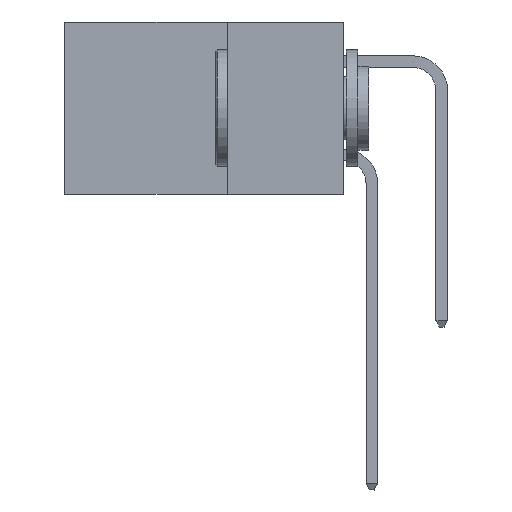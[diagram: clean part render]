
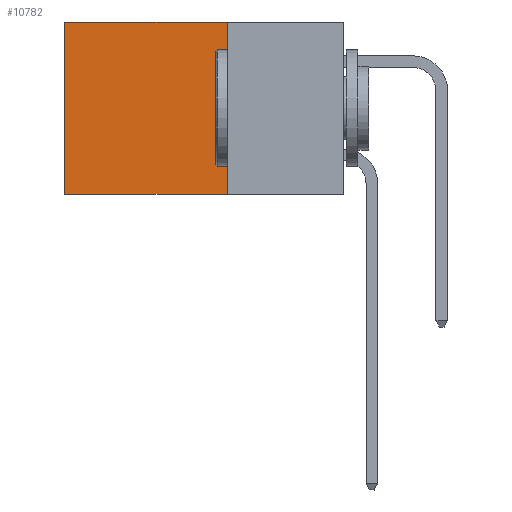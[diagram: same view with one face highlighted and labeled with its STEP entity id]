
A CAD part, left-side view. The second image highlights one B-rep face of the part: STEP entity #10782.
In plain terms, the highlighted planar face has unit normal (-1, 0, 0).
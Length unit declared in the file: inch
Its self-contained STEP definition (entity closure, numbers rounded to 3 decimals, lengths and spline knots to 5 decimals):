
#31 = ORIENTED_EDGE ( 'NONE', *, *, #5547, .F. ) ;
#980 = VERTEX_POINT ( 'NONE', #5932 ) ;
#2408 = LINE ( 'NONE', #18293, #6384 ) ;
#2844 = ORIENTED_EDGE ( 'NONE', *, *, #20150, .T. ) ;
#3345 = LINE ( 'NONE', #13109, #7808 ) ;
#3362 = DIRECTION ( 'NONE',  ( 0., 1., 0. ) ) ;
#3739 = VERTEX_POINT ( 'NONE', #16161 ) ;
#3865 = CARTESIAN_POINT ( 'NONE',  ( 0.298, 0.25, -0.37 ) ) ;
#3930 = LINE ( 'NONE', #16049, #13064 ) ;
#4838 = DIRECTION ( 'NONE',  ( 1., 0., 0. ) ) ;
#5547 = EDGE_CURVE ( 'NONE', #10440, #3739, #2408, .T. ) ;
#5686 = CARTESIAN_POINT ( 'NONE',  ( 0.298, 0.6, 0. ) ) ;
#5932 = CARTESIAN_POINT ( 'NONE',  ( 0.298, 0.25, 0. ) ) ;
#6384 = VECTOR ( 'NONE', #18337, 39.37008 ) ;
#6906 = DIRECTION ( 'NONE',  ( 0., 0., -1. ) ) ;
#7808 = VECTOR ( 'NONE', #3362, 39.37008 ) ;
#8540 = EDGE_LOOP ( 'NONE', ( #2844, #31, #13140, #15060 ) ) ;
#8905 = EDGE_CURVE ( 'NONE', #980, #10440, #3930, .T. ) ;
#9616 = VECTOR ( 'NONE', #6906, 39.37008 ) ;
#10440 = VERTEX_POINT ( 'NONE', #3865 ) ;
#10782 = ADVANCED_FACE ( 'NONE', ( #13744 ), #14467, .F. ) ;
#11275 = CARTESIAN_POINT ( 'NONE',  ( 0.298, 0.25, 0. ) ) ;
#11504 = CARTESIAN_POINT ( 'NONE',  ( 0.298, 0.6, 0. ) ) ;
#11974 = AXIS2_PLACEMENT_3D ( 'NONE', #11275, #4838, #16053 ) ;
#13064 = VECTOR ( 'NONE', #20724, 39.37008 ) ;
#13109 = CARTESIAN_POINT ( 'NONE',  ( 0.298, 0.25, 0. ) ) ;
#13140 = ORIENTED_EDGE ( 'NONE', *, *, #8905, .F. ) ;
#13744 = FACE_OUTER_BOUND ( 'NONE', #8540, .T. ) ;
#14467 = PLANE ( 'NONE',  #11974 ) ;
#15060 = ORIENTED_EDGE ( 'NONE', *, *, #16394, .T. ) ;
#16049 = CARTESIAN_POINT ( 'NONE',  ( 0.298, 0.25, 0. ) ) ;
#16053 = DIRECTION ( 'NONE',  ( 0., 0., -1. ) ) ;
#16161 = CARTESIAN_POINT ( 'NONE',  ( 0.298, 0.6, -0.37 ) ) ;
#16394 = EDGE_CURVE ( 'NONE', #980, #19398, #3345, .T. ) ;
#18019 = LINE ( 'NONE', #11504, #9616 ) ;
#18293 = CARTESIAN_POINT ( 'NONE',  ( 0.298, 0.25, -0.37 ) ) ;
#18337 = DIRECTION ( 'NONE',  ( 0., 1., 0. ) ) ;
#19398 = VERTEX_POINT ( 'NONE', #5686 ) ;
#20150 = EDGE_CURVE ( 'NONE', #19398, #3739, #18019, .T. ) ;
#20724 = DIRECTION ( 'NONE',  ( 0., 0., -1. ) ) ;
